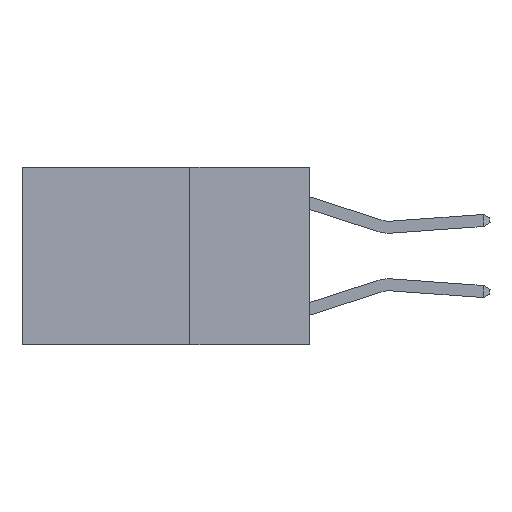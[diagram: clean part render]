
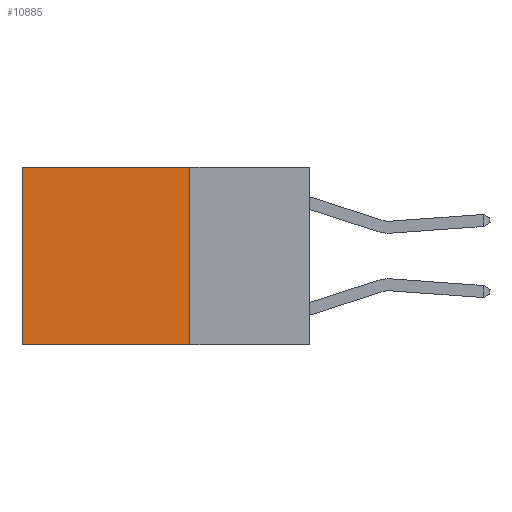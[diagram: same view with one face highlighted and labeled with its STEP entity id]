
A CAD part, left-side view. The second image highlights one B-rep face of the part: STEP entity #10885.
In plain terms, the highlighted planar face has unit normal (-1, 0, 0).
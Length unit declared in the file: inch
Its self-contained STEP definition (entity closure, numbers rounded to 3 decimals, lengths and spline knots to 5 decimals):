
#359 = CARTESIAN_POINT ( 'NONE',  ( 0.2625, 0.25, 0. ) ) ;
#471 = ORIENTED_EDGE ( 'NONE', *, *, #2003, .T. ) ;
#1186 = LINE ( 'NONE', #359, #5004 ) ;
#2003 = EDGE_CURVE ( 'NONE', #4481, #5738, #13730, .T. ) ;
#2121 = VECTOR ( 'NONE', #8020, 39.37008 ) ;
#2193 = AXIS2_PLACEMENT_3D ( 'NONE', #6613, #4480, #12616 ) ;
#2286 = FACE_OUTER_BOUND ( 'NONE', #10757, .T. ) ;
#2467 = VERTEX_POINT ( 'NONE', #9293 ) ;
#2517 = DIRECTION ( 'NONE',  ( 0., 1., 0. ) ) ;
#3323 = CARTESIAN_POINT ( 'NONE',  ( 0.2625, 0.6, 0. ) ) ;
#3753 = DIRECTION ( 'NONE',  ( 0., 0., -1. ) ) ;
#4480 = DIRECTION ( 'NONE',  ( 1., 0., 0. ) ) ;
#4481 = VERTEX_POINT ( 'NONE', #12155 ) ;
#4964 = VERTEX_POINT ( 'NONE', #13717 ) ;
#5004 = VECTOR ( 'NONE', #3753, 39.37008 ) ;
#5132 = EDGE_CURVE ( 'NONE', #4964, #2467, #1186, .T. ) ;
#5562 = PLANE ( 'NONE',  #2193 ) ;
#5738 = VERTEX_POINT ( 'NONE', #8243 ) ;
#6055 = ORIENTED_EDGE ( 'NONE', *, *, #5132, .F. ) ;
#6362 = ORIENTED_EDGE ( 'NONE', *, *, #13641, .T. ) ;
#6613 = CARTESIAN_POINT ( 'NONE',  ( 0.2625, 0.25, 0. ) ) ;
#6801 = DIRECTION ( 'NONE',  ( 0., 1., 0. ) ) ;
#6914 = EDGE_CURVE ( 'NONE', #2467, #5738, #9305, .T. ) ;
#7364 = CARTESIAN_POINT ( 'NONE',  ( 0.2625, 0.25, 0. ) ) ;
#8020 = DIRECTION ( 'NONE',  ( 0., 0., -1. ) ) ;
#8085 = CARTESIAN_POINT ( 'NONE',  ( 0.2625, 0.25, -0.37 ) ) ;
#8243 = CARTESIAN_POINT ( 'NONE',  ( 0.2625, 0.6, -0.37 ) ) ;
#9293 = CARTESIAN_POINT ( 'NONE',  ( 0.2625, 0.25, -0.37 ) ) ;
#9305 = LINE ( 'NONE', #8085, #12060 ) ;
#10757 = EDGE_LOOP ( 'NONE', ( #471, #11168, #6055, #6362 ) ) ;
#10885 = ADVANCED_FACE ( 'NONE', ( #2286 ), #5562, .F. ) ;
#11168 = ORIENTED_EDGE ( 'NONE', *, *, #6914, .F. ) ;
#11846 = LINE ( 'NONE', #7364, #13403 ) ;
#12060 = VECTOR ( 'NONE', #6801, 39.37008 ) ;
#12155 = CARTESIAN_POINT ( 'NONE',  ( 0.2625, 0.6, 0. ) ) ;
#12616 = DIRECTION ( 'NONE',  ( 0., 0., -1. ) ) ;
#13403 = VECTOR ( 'NONE', #2517, 39.37008 ) ;
#13641 = EDGE_CURVE ( 'NONE', #4964, #4481, #11846, .T. ) ;
#13717 = CARTESIAN_POINT ( 'NONE',  ( 0.2625, 0.25, 0. ) ) ;
#13730 = LINE ( 'NONE', #3323, #2121 ) ;
